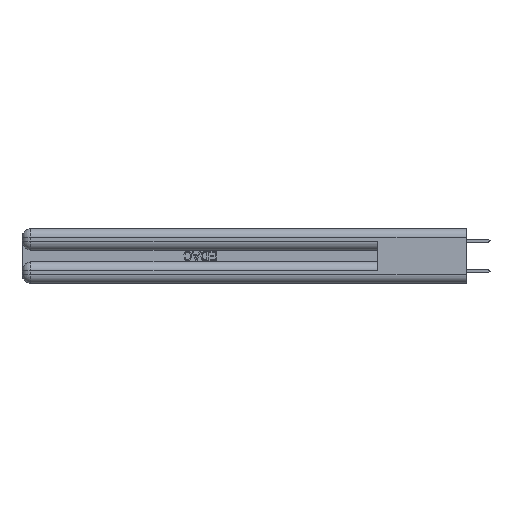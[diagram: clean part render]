
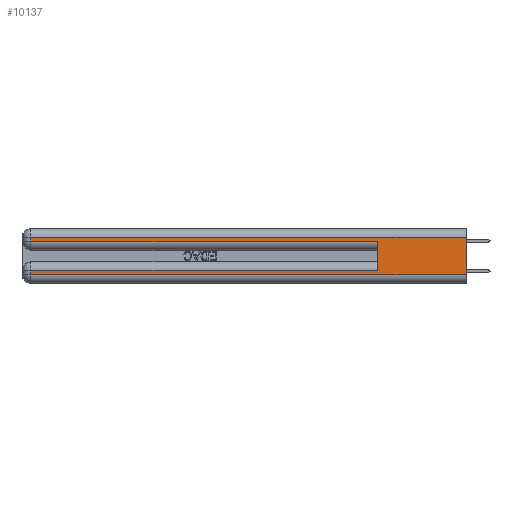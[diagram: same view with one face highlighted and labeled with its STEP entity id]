
A CAD part, left-side view. The second image highlights one B-rep face of the part: STEP entity #10137.
In plain terms, the highlighted planar face has unit normal (-1, 0, 0).
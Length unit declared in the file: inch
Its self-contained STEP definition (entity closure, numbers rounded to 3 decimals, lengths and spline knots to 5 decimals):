
#455 = CARTESIAN_POINT ( 'NONE',  ( 0., 0., 0.37 ) ) ;
#702 = DIRECTION ( 'NONE',  ( 0., 1., 0. ) ) ;
#1210 = DIRECTION ( 'NONE',  ( 0., 0., 1. ) ) ;
#1775 = VECTOR ( 'NONE', #31874, 39.37008 ) ;
#2583 = CARTESIAN_POINT ( 'NONE',  ( 0., 0., 0.31 ) ) ;
#2733 = ORIENTED_EDGE ( 'NONE', *, *, #5764, .T. ) ;
#3081 = CARTESIAN_POINT ( 'NONE',  ( 0., 2.94, 0.06 ) ) ;
#4039 = VECTOR ( 'NONE', #20971, 39.37008 ) ;
#4474 = CARTESIAN_POINT ( 'NONE',  ( 0., 0.6, 0.145 ) ) ;
#4577 = LINE ( 'NONE', #35709, #38716 ) ;
#5068 = VERTEX_POINT ( 'NONE', #17068 ) ;
#5590 = VERTEX_POINT ( 'NONE', #6069 ) ;
#5764 = EDGE_CURVE ( 'NONE', #36860, #19377, #36451, .T. ) ;
#6069 = CARTESIAN_POINT ( 'NONE',  ( 0., 0.6, 0.085 ) ) ;
#6330 = CARTESIAN_POINT ( 'NONE',  ( 0., 2.94, 0.37 ) ) ;
#7774 = CARTESIAN_POINT ( 'NONE',  ( 0., 0., 0.06 ) ) ;
#8406 = PLANE ( 'NONE',  #31774 ) ;
#8925 = LINE ( 'NONE', #6330, #44035 ) ;
#9268 = VECTOR ( 'NONE', #702, 39.37008 ) ;
#10137 = ADVANCED_FACE ( 'NONE', ( #40622 ), #8406, .F. ) ;
#10342 = EDGE_CURVE ( 'NONE', #5068, #19854, #42196, .T. ) ;
#11037 = LINE ( 'NONE', #43542, #20161 ) ;
#11881 = CARTESIAN_POINT ( 'NONE',  ( 0., 0., 0.37 ) ) ;
#13420 = EDGE_LOOP ( 'NONE', ( #18678, #2733, #24734, #27438, #25920, #43654, #14100, #19692 ) ) ;
#14100 = ORIENTED_EDGE ( 'NONE', *, *, #26016, .T. ) ;
#14558 = EDGE_CURVE ( 'NONE', #38260, #37214, #30162, .T. ) ;
#15319 = DIRECTION ( 'NONE',  ( 0., 0., -1. ) ) ;
#16391 = DIRECTION ( 'NONE',  ( 0., 1., 0. ) ) ;
#16474 = CARTESIAN_POINT ( 'NONE',  ( 0., 2.94, 0.31 ) ) ;
#17068 = CARTESIAN_POINT ( 'NONE',  ( 0., 2.94, 0.285 ) ) ;
#17766 = CARTESIAN_POINT ( 'NONE',  ( 0., 0., 0.31 ) ) ;
#18678 = ORIENTED_EDGE ( 'NONE', *, *, #19602, .F. ) ;
#18836 = LINE ( 'NONE', #4474, #19934 ) ;
#19377 = VERTEX_POINT ( 'NONE', #16474 ) ;
#19602 = EDGE_CURVE ( 'NONE', #36860, #37214, #31352, .T. ) ;
#19692 = ORIENTED_EDGE ( 'NONE', *, *, #14558, .T. ) ;
#19854 = VERTEX_POINT ( 'NONE', #29139 ) ;
#19934 = VECTOR ( 'NONE', #1210, 39.37008 ) ;
#20161 = VECTOR ( 'NONE', #16391, 39.37008 ) ;
#20593 = EDGE_CURVE ( 'NONE', #5590, #21652, #11037, .T. ) ;
#20971 = DIRECTION ( 'NONE',  ( 0., 0., -1. ) ) ;
#21620 = CARTESIAN_POINT ( 'NONE',  ( 0., 0., 0.06 ) ) ;
#21652 = VERTEX_POINT ( 'NONE', #27200 ) ;
#24172 = VECTOR ( 'NONE', #26539, 39.37008 ) ;
#24734 = ORIENTED_EDGE ( 'NONE', *, *, #38614, .T. ) ;
#25920 = ORIENTED_EDGE ( 'NONE', *, *, #34821, .F. ) ;
#26016 = EDGE_CURVE ( 'NONE', #21652, #38260, #8925, .T. ) ;
#26539 = DIRECTION ( 'NONE',  ( 0., -1., 0. ) ) ;
#27200 = CARTESIAN_POINT ( 'NONE',  ( 0., 2.94, 0.085 ) ) ;
#27438 = ORIENTED_EDGE ( 'NONE', *, *, #10342, .T. ) ;
#29139 = CARTESIAN_POINT ( 'NONE',  ( 0., 0.6, 0.285 ) ) ;
#30162 = LINE ( 'NONE', #21620, #1775 ) ;
#31352 = LINE ( 'NONE', #455, #4039 ) ;
#31774 = AXIS2_PLACEMENT_3D ( 'NONE', #11881, #35695, #15319 ) ;
#31874 = DIRECTION ( 'NONE',  ( 0., -1., 0. ) ) ;
#34821 = EDGE_CURVE ( 'NONE', #5590, #19854, #18836, .T. ) ;
#35695 = DIRECTION ( 'NONE',  ( 1., 0., 0. ) ) ;
#35709 = CARTESIAN_POINT ( 'NONE',  ( 0., 2.94, 0.37 ) ) ;
#36451 = LINE ( 'NONE', #17766, #9268 ) ;
#36860 = VERTEX_POINT ( 'NONE', #2583 ) ;
#37065 = DIRECTION ( 'NONE',  ( 0., 0., -1. ) ) ;
#37214 = VERTEX_POINT ( 'NONE', #7774 ) ;
#38260 = VERTEX_POINT ( 'NONE', #3081 ) ;
#38614 = EDGE_CURVE ( 'NONE', #19377, #5068, #4577, .T. ) ;
#38716 = VECTOR ( 'NONE', #39101, 39.37008 ) ;
#39101 = DIRECTION ( 'NONE',  ( 0., 0., -1. ) ) ;
#39965 = CARTESIAN_POINT ( 'NONE',  ( 0., 0., 0.285 ) ) ;
#40622 = FACE_OUTER_BOUND ( 'NONE', #13420, .T. ) ;
#42196 = LINE ( 'NONE', #39965, #24172 ) ;
#43542 = CARTESIAN_POINT ( 'NONE',  ( 0., 0., 0.085 ) ) ;
#43654 = ORIENTED_EDGE ( 'NONE', *, *, #20593, .T. ) ;
#44035 = VECTOR ( 'NONE', #37065, 39.37008 ) ;
